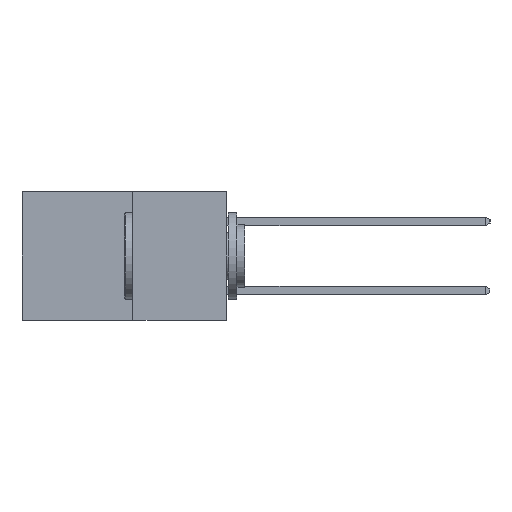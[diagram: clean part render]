
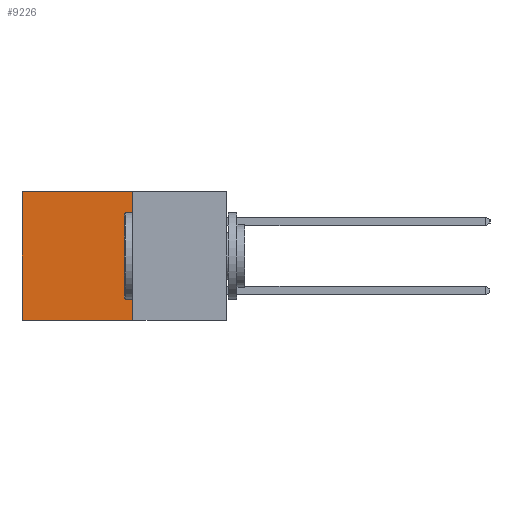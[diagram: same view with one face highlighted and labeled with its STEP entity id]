
A CAD part, left-side view. The second image highlights one B-rep face of the part: STEP entity #9226.
In plain terms, the highlighted planar face has unit normal (-1, 0, 0).
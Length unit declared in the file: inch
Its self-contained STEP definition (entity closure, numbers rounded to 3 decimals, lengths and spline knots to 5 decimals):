
#112 = VECTOR ( 'NONE', #4495, 39.37008 ) ;
#294 = CARTESIAN_POINT ( 'NONE',  ( 0.277, 0.27, -0.37 ) ) ;
#747 = EDGE_LOOP ( 'NONE', ( #5037, #11404, #5679, #5345 ) ) ;
#1038 = CARTESIAN_POINT ( 'NONE',  ( 0.277, 0.27, 0. ) ) ;
#1041 = FACE_OUTER_BOUND ( 'NONE', #747, .T. ) ;
#2275 = EDGE_CURVE ( 'NONE', #7083, #4050, #9482, .T. ) ;
#2651 = PLANE ( 'NONE',  #4803 ) ;
#3300 = LINE ( 'NONE', #294, #112 ) ;
#3686 = DIRECTION ( 'NONE',  ( 0., 0., -1. ) ) ;
#4050 = VERTEX_POINT ( 'NONE', #8193 ) ;
#4495 = DIRECTION ( 'NONE',  ( 0., 0., -1. ) ) ;
#4803 = AXIS2_PLACEMENT_3D ( 'NONE', #6775, #9943, #3686 ) ;
#4837 = DIRECTION ( 'NONE',  ( 0., 1., 0. ) ) ;
#4929 = CARTESIAN_POINT ( 'NONE',  ( 0.277, 0.27, -0.37 ) ) ;
#5037 = ORIENTED_EDGE ( 'NONE', *, *, #2275, .T. ) ;
#5345 = ORIENTED_EDGE ( 'NONE', *, *, #6652, .T. ) ;
#5679 = ORIENTED_EDGE ( 'NONE', *, *, #5790, .F. ) ;
#5790 = EDGE_CURVE ( 'NONE', #10284, #12618, #3300, .T. ) ;
#6356 = VECTOR ( 'NONE', #12193, 39.37008 ) ;
#6652 = EDGE_CURVE ( 'NONE', #10284, #7083, #12843, .T. ) ;
#6719 = EDGE_CURVE ( 'NONE', #12618, #4050, #7029, .T. ) ;
#6775 = CARTESIAN_POINT ( 'NONE',  ( 0.277, 0.27, -0.37 ) ) ;
#7029 = LINE ( 'NONE', #4929, #6356 ) ;
#7083 = VERTEX_POINT ( 'NONE', #8601 ) ;
#8193 = CARTESIAN_POINT ( 'NONE',  ( 0.277, 0.59, -0.37 ) ) ;
#8601 = CARTESIAN_POINT ( 'NONE',  ( 0.277, 0.59, 0. ) ) ;
#9128 = CARTESIAN_POINT ( 'NONE',  ( 0.277, 0.59, -0.37 ) ) ;
#9226 = ADVANCED_FACE ( 'NONE', ( #1041 ), #2651, .F. ) ;
#9482 = LINE ( 'NONE', #9128, #12534 ) ;
#9819 = VECTOR ( 'NONE', #4837, 39.37008 ) ;
#9943 = DIRECTION ( 'NONE',  ( 1., 0., 0. ) ) ;
#10284 = VERTEX_POINT ( 'NONE', #1038 ) ;
#10743 = CARTESIAN_POINT ( 'NONE',  ( 0.277, 0.27, -0.37 ) ) ;
#11404 = ORIENTED_EDGE ( 'NONE', *, *, #6719, .F. ) ;
#12106 = CARTESIAN_POINT ( 'NONE',  ( 0.277, 0.27, 0. ) ) ;
#12193 = DIRECTION ( 'NONE',  ( 0., 1., 0. ) ) ;
#12232 = DIRECTION ( 'NONE',  ( 0., 0., -1. ) ) ;
#12534 = VECTOR ( 'NONE', #12232, 39.37008 ) ;
#12618 = VERTEX_POINT ( 'NONE', #10743 ) ;
#12843 = LINE ( 'NONE', #12106, #9819 ) ;
